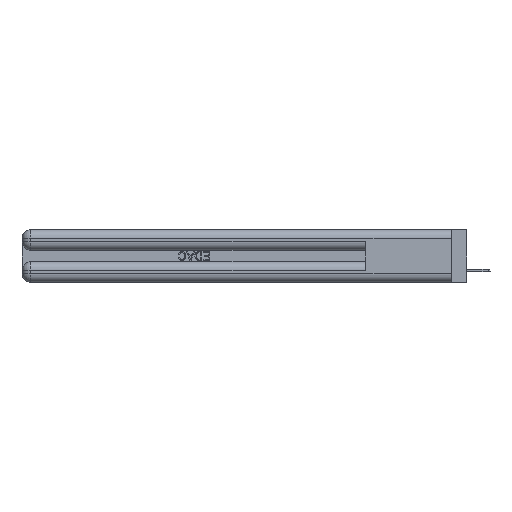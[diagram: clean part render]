
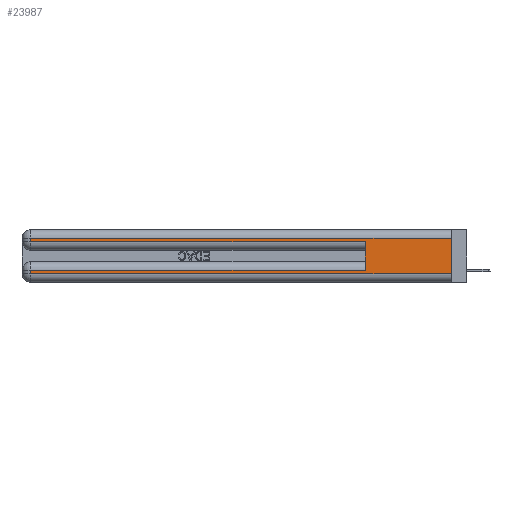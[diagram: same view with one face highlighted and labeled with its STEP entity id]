
A CAD part, left-side view. The second image highlights one B-rep face of the part: STEP entity #23987.
In plain terms, the highlighted planar face has unit normal (-1, 0, 0).
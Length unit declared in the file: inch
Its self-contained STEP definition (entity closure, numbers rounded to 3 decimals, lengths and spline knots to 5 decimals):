
#212 = VECTOR ( 'NONE', #29664, 39.37008 ) ;
#646 = LINE ( 'NONE', #45335, #19876 ) ;
#1929 = VERTEX_POINT ( 'NONE', #4208 ) ;
#2143 = EDGE_CURVE ( 'NONE', #22382, #19963, #2506, .T. ) ;
#2506 = LINE ( 'NONE', #42096, #42619 ) ;
#3180 = VECTOR ( 'NONE', #39376, 39.37008 ) ;
#4130 = LINE ( 'NONE', #15851, #44255 ) ;
#4208 = CARTESIAN_POINT ( 'NONE',  ( 0., 0.6, 0.085 ) ) ;
#5511 = LINE ( 'NONE', #9588, #3180 ) ;
#6891 = ORIENTED_EDGE ( 'NONE', *, *, #20702, .T. ) ;
#8120 = DIRECTION ( 'NONE',  ( 0., 1., 0. ) ) ;
#8469 = AXIS2_PLACEMENT_3D ( 'NONE', #43997, #29747, #25507 ) ;
#8544 = LINE ( 'NONE', #47681, #9730 ) ;
#8919 = LINE ( 'NONE', #25754, #212 ) ;
#9588 = CARTESIAN_POINT ( 'NONE',  ( 0., 0., 0.285 ) ) ;
#9730 = VECTOR ( 'NONE', #40256, 39.37008 ) ;
#11210 = ORIENTED_EDGE ( 'NONE', *, *, #27674, .T. ) ;
#12753 = CARTESIAN_POINT ( 'NONE',  ( 0., 2.94, 0.31 ) ) ;
#14320 = VERTEX_POINT ( 'NONE', #34626 ) ;
#14565 = EDGE_CURVE ( 'NONE', #33143, #14320, #8919, .T. ) ;
#14968 = DIRECTION ( 'NONE',  ( 0., 0., -1. ) ) ;
#15851 = CARTESIAN_POINT ( 'NONE',  ( 0., 0., 0.37 ) ) ;
#16798 = ORIENTED_EDGE ( 'NONE', *, *, #2143, .T. ) ;
#16983 = DIRECTION ( 'NONE',  ( 0., 0., 1. ) ) ;
#17522 = VECTOR ( 'NONE', #14968, 39.37008 ) ;
#18693 = CARTESIAN_POINT ( 'NONE',  ( 0., 2.94, 0.285 ) ) ;
#19876 = VECTOR ( 'NONE', #8120, 39.37008 ) ;
#19963 = VERTEX_POINT ( 'NONE', #18693 ) ;
#20702 = EDGE_CURVE ( 'NONE', #40159, #33143, #47762, .T. ) ;
#22382 = VERTEX_POINT ( 'NONE', #12753 ) ;
#23063 = LINE ( 'NONE', #42800, #32422 ) ;
#23845 = ORIENTED_EDGE ( 'NONE', *, *, #36796, .T. ) ;
#23890 = EDGE_CURVE ( 'NONE', #19963, #41791, #5511, .T. ) ;
#23987 = ADVANCED_FACE ( 'NONE', ( #40389 ), #40307, .F. ) ;
#25507 = DIRECTION ( 'NONE',  ( 0., 0., -1. ) ) ;
#25592 = EDGE_CURVE ( 'NONE', #28568, #14320, #4130, .T. ) ;
#25754 = CARTESIAN_POINT ( 'NONE',  ( 0., 0., 0.06 ) ) ;
#27355 = DIRECTION ( 'NONE',  ( 0., 0., -1. ) ) ;
#27674 = EDGE_CURVE ( 'NONE', #1929, #40159, #8544, .T. ) ;
#28245 = CARTESIAN_POINT ( 'NONE',  ( 0., 2.94, 0.06 ) ) ;
#28568 = VERTEX_POINT ( 'NONE', #41529 ) ;
#29511 = ORIENTED_EDGE ( 'NONE', *, *, #25592, .F. ) ;
#29655 = CARTESIAN_POINT ( 'NONE',  ( 0., 2.94, 0.37 ) ) ;
#29664 = DIRECTION ( 'NONE',  ( 0., -1., 0. ) ) ;
#29747 = DIRECTION ( 'NONE',  ( 1., 0., 0. ) ) ;
#29840 = EDGE_LOOP ( 'NONE', ( #29511, #23845, #16798, #45961, #41072, #11210, #6891, #36884 ) ) ;
#31461 = CARTESIAN_POINT ( 'NONE',  ( 0., 0.6, 0.285 ) ) ;
#32422 = VECTOR ( 'NONE', #16983, 39.37008 ) ;
#33143 = VERTEX_POINT ( 'NONE', #28245 ) ;
#34107 = DIRECTION ( 'NONE',  ( 0., 0., -1. ) ) ;
#34626 = CARTESIAN_POINT ( 'NONE',  ( 0., 0., 0.06 ) ) ;
#36796 = EDGE_CURVE ( 'NONE', #28568, #22382, #646, .T. ) ;
#36884 = ORIENTED_EDGE ( 'NONE', *, *, #14565, .T. ) ;
#39214 = CARTESIAN_POINT ( 'NONE',  ( 0., 2.94, 0.085 ) ) ;
#39376 = DIRECTION ( 'NONE',  ( 0., -1., 0. ) ) ;
#40159 = VERTEX_POINT ( 'NONE', #39214 ) ;
#40256 = DIRECTION ( 'NONE',  ( 0., 1., 0. ) ) ;
#40307 = PLANE ( 'NONE',  #8469 ) ;
#40389 = FACE_OUTER_BOUND ( 'NONE', #29840, .T. ) ;
#41072 = ORIENTED_EDGE ( 'NONE', *, *, #43716, .F. ) ;
#41529 = CARTESIAN_POINT ( 'NONE',  ( 0., 0., 0.31 ) ) ;
#41791 = VERTEX_POINT ( 'NONE', #31461 ) ;
#42096 = CARTESIAN_POINT ( 'NONE',  ( 0., 2.94, 0.37 ) ) ;
#42619 = VECTOR ( 'NONE', #27355, 39.37008 ) ;
#42800 = CARTESIAN_POINT ( 'NONE',  ( 0., 0.6, 0.145 ) ) ;
#43716 = EDGE_CURVE ( 'NONE', #1929, #41791, #23063, .T. ) ;
#43997 = CARTESIAN_POINT ( 'NONE',  ( 0., 0., 0.37 ) ) ;
#44255 = VECTOR ( 'NONE', #34107, 39.37008 ) ;
#45335 = CARTESIAN_POINT ( 'NONE',  ( 0., 0., 0.31 ) ) ;
#45961 = ORIENTED_EDGE ( 'NONE', *, *, #23890, .T. ) ;
#47681 = CARTESIAN_POINT ( 'NONE',  ( 0., 0., 0.085 ) ) ;
#47762 = LINE ( 'NONE', #29655, #17522 ) ;
